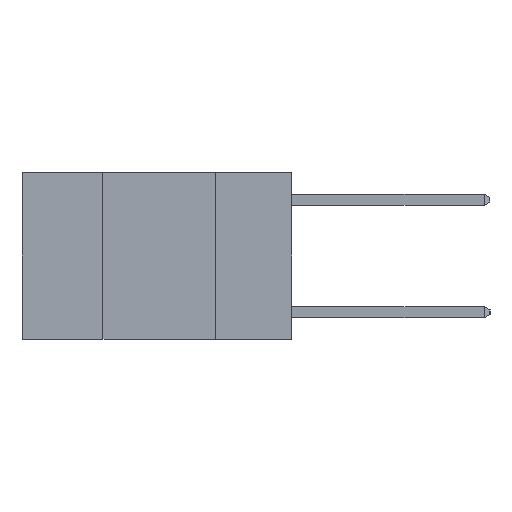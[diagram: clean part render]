
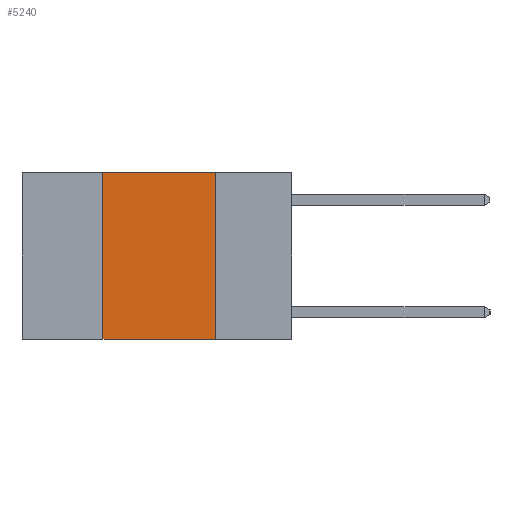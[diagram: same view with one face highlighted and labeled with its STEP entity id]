
A CAD part, left-side view. The second image highlights one B-rep face of the part: STEP entity #5240.
In plain terms, the highlighted planar face has unit normal (-1, 0, 0).
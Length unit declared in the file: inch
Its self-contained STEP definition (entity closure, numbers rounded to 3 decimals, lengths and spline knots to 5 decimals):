
#243 = CARTESIAN_POINT ( 'NONE',  ( 0., 0.42, 0. ) ) ;
#294 = VECTOR ( 'NONE', #10713, 39.37008 ) ;
#585 = LINE ( 'NONE', #6797, #2829 ) ;
#898 = ORIENTED_EDGE ( 'NONE', *, *, #1292, .F. ) ;
#982 = DIRECTION ( 'NONE',  ( 0., -1., 0. ) ) ;
#1002 = DIRECTION ( 'NONE',  ( 0., 0., -1. ) ) ;
#1292 = EDGE_CURVE ( 'NONE', #6811, #5402, #585, .T. ) ;
#1655 = CARTESIAN_POINT ( 'NONE',  ( 0., 0.6, 0. ) ) ;
#1671 = CARTESIAN_POINT ( 'NONE',  ( 0., 0.17, -0.37 ) ) ;
#1713 = FACE_OUTER_BOUND ( 'NONE', #9307, .T. ) ;
#2369 = VECTOR ( 'NONE', #1002, 39.37008 ) ;
#2497 = DIRECTION ( 'NONE',  ( 0., 0., -1. ) ) ;
#2737 = EDGE_CURVE ( 'NONE', #9945, #6811, #6909, .T. ) ;
#2829 = VECTOR ( 'NONE', #5582, 39.37008 ) ;
#2902 = AXIS2_PLACEMENT_3D ( 'NONE', #1655, #7406, #2497 ) ;
#3682 = ORIENTED_EDGE ( 'NONE', *, *, #4727, .F. ) ;
#4268 = CARTESIAN_POINT ( 'NONE',  ( 0., 0.6, -0.37 ) ) ;
#4281 = LINE ( 'NONE', #6789, #2369 ) ;
#4727 = EDGE_CURVE ( 'NONE', #5402, #10088, #4281, .T. ) ;
#5179 = CARTESIAN_POINT ( 'NONE',  ( 0., 0.17, 0. ) ) ;
#5240 = ADVANCED_FACE ( 'NONE', ( #1713 ), #10663, .F. ) ;
#5402 = VERTEX_POINT ( 'NONE', #5179 ) ;
#5582 = DIRECTION ( 'NONE',  ( 0., -1., 0. ) ) ;
#5616 = CARTESIAN_POINT ( 'NONE',  ( 0., 0.42, -0.37 ) ) ;
#6789 = CARTESIAN_POINT ( 'NONE',  ( 0., 0.17, 0. ) ) ;
#6797 = CARTESIAN_POINT ( 'NONE',  ( 0., 0.6, 0. ) ) ;
#6802 = ORIENTED_EDGE ( 'NONE', *, *, #8258, .T. ) ;
#6811 = VERTEX_POINT ( 'NONE', #9561 ) ;
#6909 = LINE ( 'NONE', #243, #294 ) ;
#7406 = DIRECTION ( 'NONE',  ( 1., 0., 0. ) ) ;
#7420 = VECTOR ( 'NONE', #982, 39.37008 ) ;
#8258 = EDGE_CURVE ( 'NONE', #9945, #10088, #9603, .T. ) ;
#9307 = EDGE_LOOP ( 'NONE', ( #3682, #898, #10326, #6802 ) ) ;
#9561 = CARTESIAN_POINT ( 'NONE',  ( 0., 0.42, 0. ) ) ;
#9603 = LINE ( 'NONE', #4268, #7420 ) ;
#9945 = VERTEX_POINT ( 'NONE', #5616 ) ;
#10088 = VERTEX_POINT ( 'NONE', #1671 ) ;
#10326 = ORIENTED_EDGE ( 'NONE', *, *, #2737, .F. ) ;
#10663 = PLANE ( 'NONE',  #2902 ) ;
#10713 = DIRECTION ( 'NONE',  ( 0., 0., 1. ) ) ;
